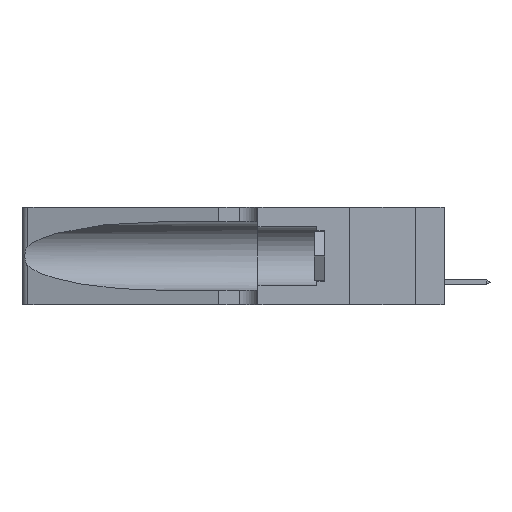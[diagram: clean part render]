
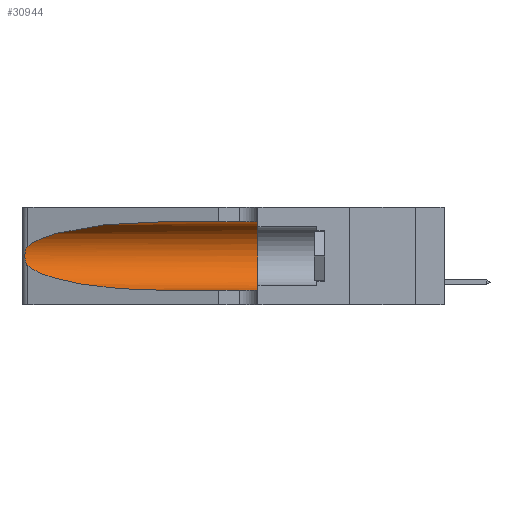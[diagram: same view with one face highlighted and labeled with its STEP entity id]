
A CAD part, left-side view. The second image highlights one B-rep face of the part: STEP entity #30944.
In plain terms, the highlighted cylindrical face has radius 3.308 mm (diameter 6.617 mm), a partial arc.
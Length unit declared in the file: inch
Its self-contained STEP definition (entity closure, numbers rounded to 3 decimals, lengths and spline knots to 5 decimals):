
#1408 = CARTESIAN_POINT ( 'NONE',  ( 0.25555, 1.22994, 0.2215 ) ) ;
#2372 = EDGE_CURVE ( 'NONE', #18980, #33992, #8665, .T. ) ;
#2986 = CIRCLE ( 'NONE', #36687, 0.13025 ) ;
#3742 = B_SPLINE_CURVE_WITH_KNOTS ( 'NONE', 3,
 ( #20701, #1408, #17032, #4182, #10620, #23880, #27022, #4777, #23437, #27152, #7812, #13821, #23586, #7974 ),
 .UNSPECIFIED., .F., .F.,
 ( 4, 2, 2, 2, 2, 2, 4 ),
 ( 0., 0.00027, 0.00053, 0.00107, 0.0016, 0.00187, 0.00214 ),
 .UNSPECIFIED. ) ;
#4011 = CARTESIAN_POINT ( 'NONE',  ( 0.25487, 1.22718, 0.22369 ) ) ;
#4182 = CARTESIAN_POINT ( 'NONE',  ( 0.25787, 1.23484, 0.2124 ) ) ;
#4458 = CARTESIAN_POINT ( 'NONE',  ( 0.1305, 0.35, 0.05475 ) ) ;
#4777 = CARTESIAN_POINT ( 'NONE',  ( 0.26075, 1.23896, 0.178 ) ) ;
#4808 = CARTESIAN_POINT ( 'NONE',  ( 0.25487, 1.22718, 0.14631 ) ) ;
#4841 = CARTESIAN_POINT ( 'NONE',  ( 0.1305, 1.61858, 0.31525 ) ) ;
#5038 = DIRECTION ( 'NONE',  ( 0., -1., 0. ) ) ;
#6913 = EDGE_CURVE ( 'NONE', #33992, #40080, #20107, .T. ) ;
#7721 = EDGE_LOOP ( 'NONE', ( #23018, #22764, #26974, #27650, #14453, #16964 ) ) ;
#7812 = CARTESIAN_POINT ( 'NONE',  ( 0.25789, 1.23486, 0.15765 ) ) ;
#7974 = CARTESIAN_POINT ( 'NONE',  ( 0.25487, 1.22718, 0.14631 ) ) ;
#8665 =( BOUNDED_CURVE ( )  B_SPLINE_CURVE ( 3, ( #40577, #9469, #37504, #31719 ),
 .UNSPECIFIED., .F., .F. ) 
 B_SPLINE_CURVE_WITH_KNOTS ( ( 4, 4 ),
 ( 3.44316, 4.71239 ),
 .UNSPECIFIED. ) 
 CURVE ( )  GEOMETRIC_REPRESENTATION_ITEM ( )  RATIONAL_B_SPLINE_CURVE ( ( 1., 0.87, 0.87, 1. ) ) 
 REPRESENTATION_ITEM ( '' )  );
#9469 = CARTESIAN_POINT ( 'NONE',  ( 0.2373, 1.15595, 0.08982 ) ) ;
#10121 = CYLINDRICAL_SURFACE ( 'NONE', #20458, 0.13025 ) ;
#10620 = CARTESIAN_POINT ( 'NONE',  ( 0.25854, 1.2359, 0.20912 ) ) ;
#10829 = LINE ( 'NONE', #4841, #14845 ) ;
#13821 = CARTESIAN_POINT ( 'NONE',  ( 0.25639, 1.23186, 0.15144 ) ) ;
#14453 = ORIENTED_EDGE ( 'NONE', *, *, #37158, .F. ) ;
#14733 = CARTESIAN_POINT ( 'NONE',  ( 0.1305, 0.35, 0.31525 ) ) ;
#14845 = VECTOR ( 'NONE', #21182, 39.37008 ) ;
#14888 = CARTESIAN_POINT ( 'NONE',  ( 0.1305, 0.35, 0.185 ) ) ;
#15384 = CARTESIAN_POINT ( 'NONE',  ( 0.1305, 1.61858, 0.185 ) ) ;
#15388 = EDGE_CURVE ( 'NONE', #35249, #17834, #10829, .T. ) ;
#16964 = ORIENTED_EDGE ( 'NONE', *, *, #15388, .F. ) ;
#17032 = CARTESIAN_POINT ( 'NONE',  ( 0.25639, 1.23184, 0.21858 ) ) ;
#17834 = VERTEX_POINT ( 'NONE', #14733 ) ;
#18346 = EDGE_CURVE ( 'NONE', #31070, #18980, #3742, .T. ) ;
#18980 = VERTEX_POINT ( 'NONE', #4808 ) ;
#20107 = LINE ( 'NONE', #25104, #22122 ) ;
#20458 = AXIS2_PLACEMENT_3D ( 'NONE', #15384, #5038, #33829 ) ;
#20644 = FACE_OUTER_BOUND ( 'NONE', #7721, .T. ) ;
#20701 = CARTESIAN_POINT ( 'NONE',  ( 0.25487, 1.22718, 0.22369 ) ) ;
#21182 = DIRECTION ( 'NONE',  ( 0., -1., 0. ) ) ;
#21475 = DIRECTION ( 'NONE',  ( 0., 1., 0. ) ) ;
#22122 = VECTOR ( 'NONE', #31935, 39.37008 ) ;
#22489 =( BOUNDED_CURVE ( )  B_SPLINE_CURVE ( 3, ( #29614, #29202, #35489, #4011 ),
 .UNSPECIFIED., .F., .T. ) 
 B_SPLINE_CURVE_WITH_KNOTS ( ( 4, 4 ),
 ( 1.5708, 2.84003 ),
 .UNSPECIFIED. ) 
 CURVE ( )  GEOMETRIC_REPRESENTATION_ITEM ( )  RATIONAL_B_SPLINE_CURVE ( ( 1., 0.87, 0.87, 1. ) ) 
 REPRESENTATION_ITEM ( '' )  );
#22764 = ORIENTED_EDGE ( 'NONE', *, *, #18346, .T. ) ;
#23018 = ORIENTED_EDGE ( 'NONE', *, *, #38035, .T. ) ;
#23437 = CARTESIAN_POINT ( 'NONE',  ( 0.26017, 1.23833, 0.17102 ) ) ;
#23586 = CARTESIAN_POINT ( 'NONE',  ( 0.25555, 1.22993, 0.14849 ) ) ;
#23880 = CARTESIAN_POINT ( 'NONE',  ( 0.26018, 1.23835, 0.19895 ) ) ;
#25104 = CARTESIAN_POINT ( 'NONE',  ( 0.1305, 1.61858, 0.05475 ) ) ;
#26974 = ORIENTED_EDGE ( 'NONE', *, *, #2372, .T. ) ;
#27022 = CARTESIAN_POINT ( 'NONE',  ( 0.26075, 1.23896, 0.19203 ) ) ;
#27152 = CARTESIAN_POINT ( 'NONE',  ( 0.25856, 1.23593, 0.16098 ) ) ;
#27650 = ORIENTED_EDGE ( 'NONE', *, *, #6913, .T. ) ;
#27864 = CARTESIAN_POINT ( 'NONE',  ( 0.1305, 0.72297, 0.31525 ) ) ;
#29202 = CARTESIAN_POINT ( 'NONE',  ( 0.18966, 0.96281, 0.31525 ) ) ;
#29614 = CARTESIAN_POINT ( 'NONE',  ( 0.1305, 0.72297, 0.31525 ) ) ;
#30944 = ADVANCED_FACE ( 'NONE', ( #20644 ), #10121, .F. ) ;
#31070 = VERTEX_POINT ( 'NONE', #33519 ) ;
#31719 = CARTESIAN_POINT ( 'NONE',  ( 0.1305, 0.72297, 0.05475 ) ) ;
#31935 = DIRECTION ( 'NONE',  ( 0., -1., 0. ) ) ;
#33519 = CARTESIAN_POINT ( 'NONE',  ( 0.25487, 1.22718, 0.22369 ) ) ;
#33829 = DIRECTION ( 'NONE',  ( 0., 0., -1. ) ) ;
#33992 = VERTEX_POINT ( 'NONE', #39745 ) ;
#34198 = DIRECTION ( 'NONE',  ( 0., 0., 1. ) ) ;
#35249 = VERTEX_POINT ( 'NONE', #27864 ) ;
#35489 = CARTESIAN_POINT ( 'NONE',  ( 0.2373, 1.15595, 0.28018 ) ) ;
#36687 = AXIS2_PLACEMENT_3D ( 'NONE', #14888, #21475, #34198 ) ;
#37158 = EDGE_CURVE ( 'NONE', #17834, #40080, #2986, .T. ) ;
#37504 = CARTESIAN_POINT ( 'NONE',  ( 0.18966, 0.96281, 0.05475 ) ) ;
#38035 = EDGE_CURVE ( 'NONE', #35249, #31070, #22489, .T. ) ;
#39745 = CARTESIAN_POINT ( 'NONE',  ( 0.1305, 0.72297, 0.05475 ) ) ;
#40080 = VERTEX_POINT ( 'NONE', #4458 ) ;
#40577 = CARTESIAN_POINT ( 'NONE',  ( 0.25487, 1.22718, 0.14631 ) ) ;
